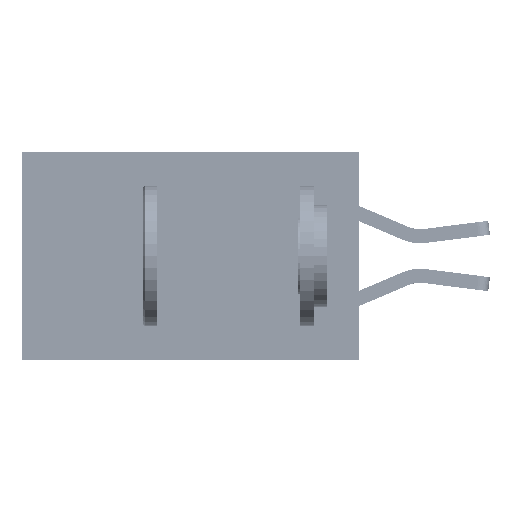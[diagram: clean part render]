
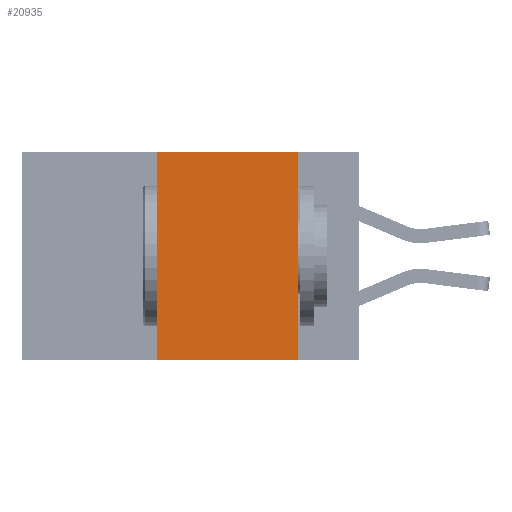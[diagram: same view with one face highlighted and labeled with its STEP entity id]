
A CAD part, left-side view. The second image highlights one B-rep face of the part: STEP entity #20935.
In plain terms, the highlighted planar face has unit normal (-1, 0, 0).
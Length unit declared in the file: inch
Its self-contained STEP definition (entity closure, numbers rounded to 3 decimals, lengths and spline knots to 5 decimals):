
#1087 = EDGE_CURVE ( 'NONE', #9207, #43899, #19399, .T. ) ;
#2157 = PLANE ( 'NONE',  #11818 ) ;
#5378 = ORIENTED_EDGE ( 'NONE', *, *, #36643, .F. ) ;
#6319 = DIRECTION ( 'NONE',  ( 0., 0., -1. ) ) ;
#9207 = VERTEX_POINT ( 'NONE', #39243 ) ;
#9614 = CARTESIAN_POINT ( 'NONE',  ( 0., 0.6, -0.37 ) ) ;
#11467 = CARTESIAN_POINT ( 'NONE',  ( 0., 0.11, 0. ) ) ;
#11509 = CARTESIAN_POINT ( 'NONE',  ( 0., 0.6, 0. ) ) ;
#11818 = AXIS2_PLACEMENT_3D ( 'NONE', #14450, #30875, #6319 ) ;
#11868 = ORIENTED_EDGE ( 'NONE', *, *, #22715, .F. ) ;
#14301 = CARTESIAN_POINT ( 'NONE',  ( 0., 0.36, -0.37 ) ) ;
#14450 = CARTESIAN_POINT ( 'NONE',  ( 0., 0.6, 0. ) ) ;
#15907 = FACE_OUTER_BOUND ( 'NONE', #23515, .T. ) ;
#17576 = CARTESIAN_POINT ( 'NONE',  ( 0., 0.11, -0.37 ) ) ;
#19399 = LINE ( 'NONE', #11509, #30258 ) ;
#19994 = VECTOR ( 'NONE', #34852, 39.37008 ) ;
#20935 = ADVANCED_FACE ( 'NONE', ( #15907 ), #2157, .F. ) ;
#22715 = EDGE_CURVE ( 'NONE', #43899, #43575, #30866, .T. ) ;
#23264 = LINE ( 'NONE', #9614, #35372 ) ;
#23515 = EDGE_LOOP ( 'NONE', ( #11868, #39917, #5378, #33593 ) ) ;
#27151 = CARTESIAN_POINT ( 'NONE',  ( 0., 0.36, 0. ) ) ;
#27790 = DIRECTION ( 'NONE',  ( 0., -1., 0. ) ) ;
#30258 = VECTOR ( 'NONE', #27790, 39.37008 ) ;
#30866 = LINE ( 'NONE', #38903, #19994 ) ;
#30875 = DIRECTION ( 'NONE',  ( 1., 0., 0. ) ) ;
#31935 = DIRECTION ( 'NONE',  ( 0., 0., 1. ) ) ;
#33593 = ORIENTED_EDGE ( 'NONE', *, *, #51946, .T. ) ;
#34852 = DIRECTION ( 'NONE',  ( 0., 0., -1. ) ) ;
#35372 = VECTOR ( 'NONE', #50225, 39.37008 ) ;
#36643 = EDGE_CURVE ( 'NONE', #41230, #9207, #49714, .T. ) ;
#38903 = CARTESIAN_POINT ( 'NONE',  ( 0., 0.11, 0. ) ) ;
#38927 = VECTOR ( 'NONE', #31935, 39.37008 ) ;
#39243 = CARTESIAN_POINT ( 'NONE',  ( 0., 0.36, 0. ) ) ;
#39917 = ORIENTED_EDGE ( 'NONE', *, *, #1087, .F. ) ;
#41230 = VERTEX_POINT ( 'NONE', #14301 ) ;
#43575 = VERTEX_POINT ( 'NONE', #17576 ) ;
#43899 = VERTEX_POINT ( 'NONE', #11467 ) ;
#49714 = LINE ( 'NONE', #27151, #38927 ) ;
#50225 = DIRECTION ( 'NONE',  ( 0., -1., 0. ) ) ;
#51946 = EDGE_CURVE ( 'NONE', #41230, #43575, #23264, .T. ) ;
